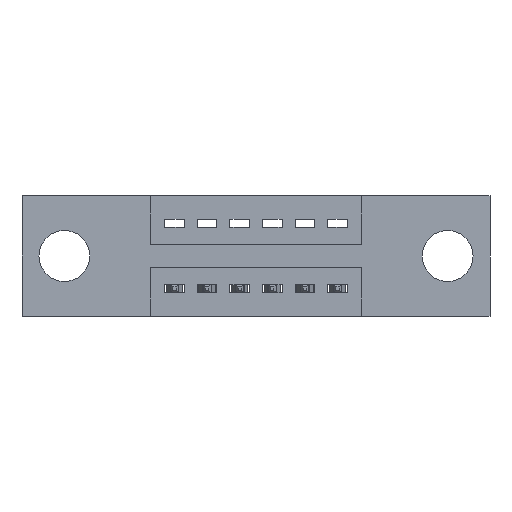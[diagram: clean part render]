
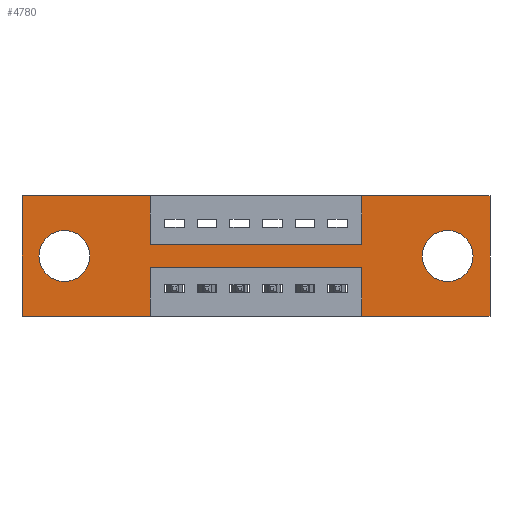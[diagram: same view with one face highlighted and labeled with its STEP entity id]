
A CAD part, front view. The second image highlights one B-rep face of the part: STEP entity #4780.
In plain terms, the highlighted planar face has unit normal (0, -1, 0).
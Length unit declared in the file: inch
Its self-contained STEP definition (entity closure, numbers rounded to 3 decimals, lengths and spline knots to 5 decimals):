
#294 = FACE_BOUND ( 'NONE', #4337, .T. ) ;
#327 = EDGE_CURVE ( 'NONE', #8765, #2852, #4909, .T. ) ;
#339 = EDGE_CURVE ( 'NONE', #4626, #8515, #9389, .T. ) ;
#367 = VECTOR ( 'NONE', #9217, 39.37008 ) ;
#488 = CARTESIAN_POINT ( 'NONE',  ( 1.435, 0., 0. ) ) ;
#550 = VECTOR ( 'NONE', #4706, 39.37008 ) ;
#596 = LINE ( 'NONE', #5562, #9126 ) ;
#861 = DIRECTION ( 'NONE',  ( 0., 0., -1. ) ) ;
#922 = DIRECTION ( 'NONE',  ( 1., 0., 0. ) ) ;
#996 = EDGE_CURVE ( 'NONE', #4612, #3359, #596, .T. ) ;
#1057 = VERTEX_POINT ( 'NONE', #4993 ) ;
#1078 = CARTESIAN_POINT ( 'NONE',  ( 0.3925, 0., 0. ) ) ;
#1131 = LINE ( 'NONE', #2343, #8645 ) ;
#1278 = EDGE_CURVE ( 'NONE', #1846, #2486, #2058, .T. ) ;
#1465 = VERTEX_POINT ( 'NONE', #6270 ) ;
#1607 = CARTESIAN_POINT ( 'NONE',  ( 0., 0., 0. ) ) ;
#1633 = DIRECTION ( 'NONE',  ( 0., 0., -1. ) ) ;
#1663 = DIRECTION ( 'NONE',  ( 0., -1., 0. ) ) ;
#1676 = ORIENTED_EDGE ( 'NONE', *, *, #9130, .F. ) ;
#1705 = VECTOR ( 'NONE', #8503, 39.37008 ) ;
#1734 = PLANE ( 'NONE',  #1768 ) ;
#1749 = CARTESIAN_POINT ( 'NONE',  ( 1.305, 0., -0.185 ) ) ;
#1761 = CARTESIAN_POINT ( 'NONE',  ( 0., 0., -0.37 ) ) ;
#1768 = AXIS2_PLACEMENT_3D ( 'NONE', #3868, #1663, #8945 ) ;
#1773 = DIRECTION ( 'NONE',  ( -1., 0., 0. ) ) ;
#1846 = VERTEX_POINT ( 'NONE', #6830 ) ;
#1936 = VERTEX_POINT ( 'NONE', #7791 ) ;
#1981 = EDGE_CURVE ( 'NONE', #8515, #1057, #8949, .T. ) ;
#2058 = LINE ( 'NONE', #1607, #7661 ) ;
#2161 = ORIENTED_EDGE ( 'NONE', *, *, #3981, .F. ) ;
#2260 = CIRCLE ( 'NONE', #6294, 0.078 ) ;
#2343 = CARTESIAN_POINT ( 'NONE',  ( 1.0425, 0., -0.37 ) ) ;
#2486 = VERTEX_POINT ( 'NONE', #9056 ) ;
#2539 = DIRECTION ( 'NONE',  ( -1., 0., 0. ) ) ;
#2692 = ORIENTED_EDGE ( 'NONE', *, *, #1278, .F. ) ;
#2777 = CARTESIAN_POINT ( 'NONE',  ( 0., 0., 0. ) ) ;
#2846 = CARTESIAN_POINT ( 'NONE',  ( 0.3925, 0., 0. ) ) ;
#2852 = VERTEX_POINT ( 'NONE', #7492 ) ;
#2876 = AXIS2_PLACEMENT_3D ( 'NONE', #6729, #6001, #861 ) ;
#2884 = EDGE_CURVE ( 'NONE', #4856, #7411, #2260, .T. ) ;
#2991 = ORIENTED_EDGE ( 'NONE', *, *, #5156, .F. ) ;
#3090 = ORIENTED_EDGE ( 'NONE', *, *, #2884, .T. ) ;
#3138 = VECTOR ( 'NONE', #7611, 39.37008 ) ;
#3185 = VECTOR ( 'NONE', #1633, 39.37008 ) ;
#3194 = CIRCLE ( 'NONE', #6072, 0.078 ) ;
#3309 = CARTESIAN_POINT ( 'NONE',  ( 0.3925, 0., -0.22 ) ) ;
#3359 = VERTEX_POINT ( 'NONE', #9306 ) ;
#3469 = DIRECTION ( 'NONE',  ( 0., 1., 0. ) ) ;
#3858 = DIRECTION ( 'NONE',  ( 0., 0., 1. ) ) ;
#3868 = CARTESIAN_POINT ( 'NONE',  ( 0., 0., -0.37 ) ) ;
#3981 = EDGE_CURVE ( 'NONE', #1936, #8833, #8238, .T. ) ;
#4056 = ORIENTED_EDGE ( 'NONE', *, *, #8371, .F. ) ;
#4069 = ORIENTED_EDGE ( 'NONE', *, *, #339, .F. ) ;
#4331 = DIRECTION ( 'NONE',  ( 0., 1., 0. ) ) ;
#4337 = EDGE_LOOP ( 'NONE', ( #8815, #3090 ) ) ;
#4345 = CARTESIAN_POINT ( 'NONE',  ( 0.3925, 0., -0.22 ) ) ;
#4389 = EDGE_CURVE ( 'NONE', #1465, #6330, #4653, .T. ) ;
#4558 = CARTESIAN_POINT ( 'NONE',  ( 0.3925, 0., -0.37 ) ) ;
#4612 = VERTEX_POINT ( 'NONE', #6818 ) ;
#4626 = VERTEX_POINT ( 'NONE', #7581 ) ;
#4653 = CIRCLE ( 'NONE', #4738, 0.078 ) ;
#4674 = VECTOR ( 'NONE', #6123, 39.37008 ) ;
#4706 = DIRECTION ( 'NONE',  ( 0., 0., 1. ) ) ;
#4720 = DIRECTION ( 'NONE',  ( 0., 0., 1. ) ) ;
#4723 = DIRECTION ( 'NONE',  ( 0., 1., 0. ) ) ;
#4738 = AXIS2_PLACEMENT_3D ( 'NONE', #1749, #3469, #6457 ) ;
#4780 = ADVANCED_FACE ( 'NONE', ( #6420, #294, #7674 ), #1734, .T. ) ;
#4856 = VERTEX_POINT ( 'NONE', #7101 ) ;
#4901 = VECTOR ( 'NONE', #5067, 39.37008 ) ;
#4909 = LINE ( 'NONE', #1078, #4674 ) ;
#4993 = CARTESIAN_POINT ( 'NONE',  ( 0., 0., 0. ) ) ;
#5067 = DIRECTION ( 'NONE',  ( 0., 0., 1. ) ) ;
#5075 = EDGE_CURVE ( 'NONE', #6330, #1465, #6250, .T. ) ;
#5098 = CARTESIAN_POINT ( 'NONE',  ( 0.13, 0., -0.107 ) ) ;
#5115 = DIRECTION ( 'NONE',  ( 0., 0., 1. ) ) ;
#5156 = EDGE_CURVE ( 'NONE', #5614, #1846, #6257, .T. ) ;
#5307 = ORIENTED_EDGE ( 'NONE', *, *, #4389, .T. ) ;
#5562 = CARTESIAN_POINT ( 'NONE',  ( 0., 0., -0.37 ) ) ;
#5614 = VERTEX_POINT ( 'NONE', #6556 ) ;
#5777 = CARTESIAN_POINT ( 'NONE',  ( 0.13, 0., -0.185 ) ) ;
#5834 = EDGE_CURVE ( 'NONE', #8833, #4626, #7637, .T. ) ;
#5946 = ORIENTED_EDGE ( 'NONE', *, *, #6505, .F. ) ;
#6001 = DIRECTION ( 'NONE',  ( 0., 1., 0. ) ) ;
#6072 = AXIS2_PLACEMENT_3D ( 'NONE', #5777, #4331, #5115 ) ;
#6123 = DIRECTION ( 'NONE',  ( 0., 0., -1. ) ) ;
#6151 = LINE ( 'NONE', #488, #367 ) ;
#6250 = CIRCLE ( 'NONE', #2876, 0.078 ) ;
#6257 = LINE ( 'NONE', #7585, #550 ) ;
#6270 = CARTESIAN_POINT ( 'NONE',  ( 1.305, 0., -0.107 ) ) ;
#6294 = AXIS2_PLACEMENT_3D ( 'NONE', #9040, #4723, #3858 ) ;
#6298 = VECTOR ( 'NONE', #2539, 39.37008 ) ;
#6330 = VERTEX_POINT ( 'NONE', #8914 ) ;
#6420 = FACE_BOUND ( 'NONE', #7827, .T. ) ;
#6457 = DIRECTION ( 'NONE',  ( 0., 0., -1. ) ) ;
#6480 = ORIENTED_EDGE ( 'NONE', *, *, #1981, .F. ) ;
#6505 = EDGE_CURVE ( 'NONE', #1057, #8765, #8990, .T. ) ;
#6549 = EDGE_CURVE ( 'NONE', #7411, #4856, #3194, .T. ) ;
#6556 = CARTESIAN_POINT ( 'NONE',  ( 1.0425, 0., -0.15 ) ) ;
#6658 = EDGE_LOOP ( 'NONE', ( #7256, #2161, #8870, #6760, #4056, #2692, #2991, #1676, #8092, #5946, #6480, #4069 ) ) ;
#6673 = ORIENTED_EDGE ( 'NONE', *, *, #5075, .T. ) ;
#6729 = CARTESIAN_POINT ( 'NONE',  ( 1.305, 0., -0.185 ) ) ;
#6760 = ORIENTED_EDGE ( 'NONE', *, *, #996, .F. ) ;
#6818 = CARTESIAN_POINT ( 'NONE',  ( 1.435, 0., -0.37 ) ) ;
#6830 = CARTESIAN_POINT ( 'NONE',  ( 1.0425, 0., 0. ) ) ;
#6914 = DIRECTION ( 'NONE',  ( 1., 0., 0. ) ) ;
#6985 = CARTESIAN_POINT ( 'NONE',  ( 0., 0., -0.37 ) ) ;
#7101 = CARTESIAN_POINT ( 'NONE',  ( 0.13, 0., -0.263 ) ) ;
#7113 = EDGE_CURVE ( 'NONE', #3359, #1936, #1131, .T. ) ;
#7256 = ORIENTED_EDGE ( 'NONE', *, *, #5834, .F. ) ;
#7411 = VERTEX_POINT ( 'NONE', #5098 ) ;
#7492 = CARTESIAN_POINT ( 'NONE',  ( 0.3925, 0., -0.15 ) ) ;
#7504 = VECTOR ( 'NONE', #6914, 39.37008 ) ;
#7581 = CARTESIAN_POINT ( 'NONE',  ( 0.3925, 0., -0.37 ) ) ;
#7585 = CARTESIAN_POINT ( 'NONE',  ( 1.0425, 0., 0. ) ) ;
#7611 = DIRECTION ( 'NONE',  ( -1., 0., 0. ) ) ;
#7637 = LINE ( 'NONE', #4558, #3185 ) ;
#7661 = VECTOR ( 'NONE', #922, 39.37008 ) ;
#7674 = FACE_OUTER_BOUND ( 'NONE', #6658, .T. ) ;
#7791 = CARTESIAN_POINT ( 'NONE',  ( 1.0425, 0., -0.22 ) ) ;
#7827 = EDGE_LOOP ( 'NONE', ( #5307, #6673 ) ) ;
#8092 = ORIENTED_EDGE ( 'NONE', *, *, #327, .F. ) ;
#8238 = LINE ( 'NONE', #3309, #6298 ) ;
#8371 = EDGE_CURVE ( 'NONE', #2486, #4612, #6151, .T. ) ;
#8387 = CARTESIAN_POINT ( 'NONE',  ( 0.3925, 0., -0.15 ) ) ;
#8430 = LINE ( 'NONE', #8387, #7504 ) ;
#8503 = DIRECTION ( 'NONE',  ( 1., 0., 0. ) ) ;
#8515 = VERTEX_POINT ( 'NONE', #1761 ) ;
#8645 = VECTOR ( 'NONE', #4720, 39.37008 ) ;
#8765 = VERTEX_POINT ( 'NONE', #2846 ) ;
#8815 = ORIENTED_EDGE ( 'NONE', *, *, #6549, .T. ) ;
#8833 = VERTEX_POINT ( 'NONE', #4345 ) ;
#8870 = ORIENTED_EDGE ( 'NONE', *, *, #7113, .F. ) ;
#8914 = CARTESIAN_POINT ( 'NONE',  ( 1.305, 0., -0.263 ) ) ;
#8945 = DIRECTION ( 'NONE',  ( 0., 0., -1. ) ) ;
#8949 = LINE ( 'NONE', #2777, #4901 ) ;
#8990 = LINE ( 'NONE', #9262, #1705 ) ;
#9040 = CARTESIAN_POINT ( 'NONE',  ( 0.13, 0., -0.185 ) ) ;
#9056 = CARTESIAN_POINT ( 'NONE',  ( 1.435, 0., 0. ) ) ;
#9126 = VECTOR ( 'NONE', #1773, 39.37008 ) ;
#9130 = EDGE_CURVE ( 'NONE', #2852, #5614, #8430, .T. ) ;
#9217 = DIRECTION ( 'NONE',  ( 0., 0., -1. ) ) ;
#9262 = CARTESIAN_POINT ( 'NONE',  ( 0., 0., 0. ) ) ;
#9306 = CARTESIAN_POINT ( 'NONE',  ( 1.0425, 0., -0.37 ) ) ;
#9389 = LINE ( 'NONE', #6985, #3138 ) ;
